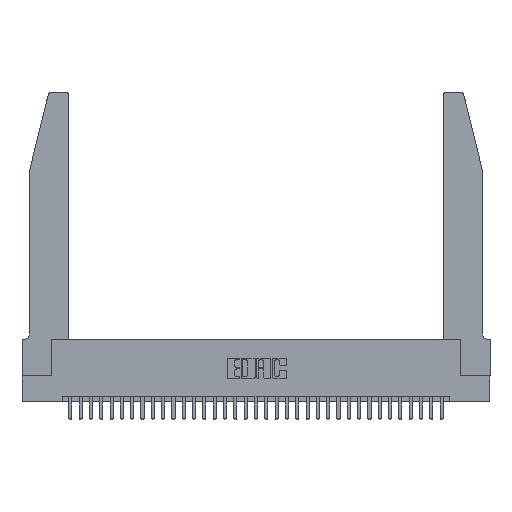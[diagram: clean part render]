
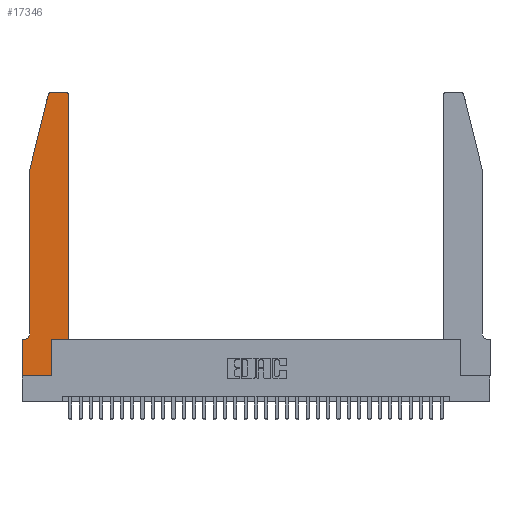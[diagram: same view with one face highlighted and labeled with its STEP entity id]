
A CAD part, top view. The second image highlights one B-rep face of the part: STEP entity #17346.
In plain terms, the highlighted planar face has unit normal (0, 0, 1).
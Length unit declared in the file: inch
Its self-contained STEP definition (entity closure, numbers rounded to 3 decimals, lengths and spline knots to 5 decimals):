
#18 = LINE ( 'NONE', #7296, #27140 ) ;
#50 = AXIS2_PLACEMENT_3D ( 'NONE', #32240, #16241, #21627 ) ;
#157 = CARTESIAN_POINT ( 'NONE',  ( 0.4505, 2.72, 0.37 ) ) ;
#393 = EDGE_LOOP ( 'NONE', ( #25358, #10739, #2610, #29178, #9738, #2797, #30110, #21953, #15608, #13104, #11026, #16467 ) ) ;
#532 = CARTESIAN_POINT ( 'NONE',  ( 0., 0., 0.37 ) ) ;
#1528 = CARTESIAN_POINT ( 'NONE',  ( 0.4205, 2.75, 0.37 ) ) ;
#1708 = EDGE_CURVE ( 'NONE', #29478, #9173, #33890, .T. ) ;
#2610 = ORIENTED_EDGE ( 'NONE', *, *, #3588, .T. ) ;
#2797 = ORIENTED_EDGE ( 'NONE', *, *, #6301, .T. ) ;
#2839 = VECTOR ( 'NONE', #18479, 39.37008 ) ;
#3296 = VECTOR ( 'NONE', #26003, 39.37008 ) ;
#3483 = EDGE_CURVE ( 'NONE', #32166, #7659, #15396, .T. ) ;
#3588 = EDGE_CURVE ( 'NONE', #21038, #27131, #17915, .T. ) ;
#3606 = VERTEX_POINT ( 'NONE', #157 ) ;
#3608 = DIRECTION ( 'NONE',  ( 1., 0., 0. ) ) ;
#3893 = CARTESIAN_POINT ( 'NONE',  ( 0.4505, 0.35, 0.37 ) ) ;
#5237 = AXIS2_PLACEMENT_3D ( 'NONE', #26455, #20796, #34541 ) ;
#5269 = CIRCLE ( 'NONE', #12655, 0.03 ) ;
#6301 = EDGE_CURVE ( 'NONE', #30680, #23756, #9746, .T. ) ;
#6349 = PLANE ( 'NONE',  #9147 ) ;
#7296 = CARTESIAN_POINT ( 'NONE',  ( 0., 0., 0.37 ) ) ;
#7659 = VERTEX_POINT ( 'NONE', #31072 ) ;
#8230 = LINE ( 'NONE', #12287, #31274 ) ;
#8306 = LINE ( 'NONE', #33399, #21710 ) ;
#8800 = EDGE_CURVE ( 'NONE', #9173, #21038, #5269, .T. ) ;
#9147 = AXIS2_PLACEMENT_3D ( 'NONE', #22483, #11845, #14546 ) ;
#9173 = VERTEX_POINT ( 'NONE', #15571 ) ;
#9477 = CARTESIAN_POINT ( 'NONE',  ( 0.0755, 2., 0.37 ) ) ;
#9738 = ORIENTED_EDGE ( 'NONE', *, *, #21469, .T. ) ;
#9746 = LINE ( 'NONE', #30534, #12687 ) ;
#9752 = CARTESIAN_POINT ( 'NONE',  ( 0.2865, 0.35, 0.37 ) ) ;
#10739 = ORIENTED_EDGE ( 'NONE', *, *, #8800, .T. ) ;
#10910 = CIRCLE ( 'NONE', #50, 0.03 ) ;
#10980 = CARTESIAN_POINT ( 'NONE',  ( 0.0755, 0.42, 0.37 ) ) ;
#11026 = ORIENTED_EDGE ( 'NONE', *, *, #15504, .T. ) ;
#11180 = CARTESIAN_POINT ( 'NONE',  ( 0.4505, 0.35, 0.37 ) ) ;
#11372 = LINE ( 'NONE', #11180, #33586 ) ;
#11845 = DIRECTION ( 'NONE',  ( 0., 0., 1. ) ) ;
#12050 = DIRECTION ( 'NONE',  ( 0., -1., 0. ) ) ;
#12287 = CARTESIAN_POINT ( 'NONE',  ( 0.0755, 2., 0.37 ) ) ;
#12655 = AXIS2_PLACEMENT_3D ( 'NONE', #27815, #22693, #22561 ) ;
#12687 = VECTOR ( 'NONE', #32031, 39.37008 ) ;
#12818 = EDGE_CURVE ( 'NONE', #23756, #34601, #18, .T. ) ;
#13095 = CARTESIAN_POINT ( 'NONE',  ( 0.2865, 0., 0.37 ) ) ;
#13104 = ORIENTED_EDGE ( 'NONE', *, *, #18372, .T. ) ;
#14381 = FACE_OUTER_BOUND ( 'NONE', #393, .T. ) ;
#14546 = DIRECTION ( 'NONE',  ( 1., 0., 0. ) ) ;
#15038 = EDGE_CURVE ( 'NONE', #34601, #32166, #8306, .T. ) ;
#15396 = LINE ( 'NONE', #9752, #17459 ) ;
#15504 = EDGE_CURVE ( 'NONE', #23414, #3606, #16597, .T. ) ;
#15571 = CARTESIAN_POINT ( 'NONE',  ( 0.284, 2.75, 0.37 ) ) ;
#15608 = ORIENTED_EDGE ( 'NONE', *, *, #3483, .T. ) ;
#16241 = DIRECTION ( 'NONE',  ( 0., 0., 1. ) ) ;
#16467 = ORIENTED_EDGE ( 'NONE', *, *, #32716, .T. ) ;
#16597 = LINE ( 'NONE', #3893, #34224 ) ;
#17217 = CARTESIAN_POINT ( 'NONE',  ( 0.25487, 2.72718, 0.37 ) ) ;
#17346 = ADVANCED_FACE ( 'NONE', ( #14381 ), #6349, .T. ) ;
#17459 = VECTOR ( 'NONE', #25511, 39.37008 ) ;
#17915 = LINE ( 'NONE', #34373, #2839 ) ;
#18372 = EDGE_CURVE ( 'NONE', #7659, #23414, #11372, .T. ) ;
#18479 = DIRECTION ( 'NONE',  ( -0.239, -0.971, 0. ) ) ;
#19720 = CARTESIAN_POINT ( 'NONE',  ( 0.0055, 0.35, 0.37 ) ) ;
#20796 = DIRECTION ( 'NONE',  ( 0., 0., -1. ) ) ;
#21038 = VERTEX_POINT ( 'NONE', #17217 ) ;
#21469 = EDGE_CURVE ( 'NONE', #29956, #30680, #31533, .T. ) ;
#21627 = DIRECTION ( 'NONE',  ( 1., 0., 0. ) ) ;
#21710 = VECTOR ( 'NONE', #28636, 39.37008 ) ;
#21931 = CARTESIAN_POINT ( 'NONE',  ( 0.4505, 0.35, 0.37 ) ) ;
#21953 = ORIENTED_EDGE ( 'NONE', *, *, #15038, .T. ) ;
#22483 = CARTESIAN_POINT ( 'NONE',  ( 0., 0.35, 0.37 ) ) ;
#22561 = DIRECTION ( 'NONE',  ( 1., 0., 0. ) ) ;
#22693 = DIRECTION ( 'NONE',  ( 0., 0., 1. ) ) ;
#23414 = VERTEX_POINT ( 'NONE', #21931 ) ;
#23576 = CARTESIAN_POINT ( 'NONE',  ( 0.2605, 2.75, 0.37 ) ) ;
#23756 = VERTEX_POINT ( 'NONE', #27217 ) ;
#25247 = DIRECTION ( 'NONE',  ( 0., 1., 0. ) ) ;
#25358 = ORIENTED_EDGE ( 'NONE', *, *, #1708, .T. ) ;
#25511 = DIRECTION ( 'NONE',  ( 0., 1., 0. ) ) ;
#25781 = EDGE_CURVE ( 'NONE', #27131, #29956, #8230, .T. ) ;
#26003 = DIRECTION ( 'NONE',  ( -1., 0., 0. ) ) ;
#26162 = DIRECTION ( 'NONE',  ( 0., -1., 0. ) ) ;
#26455 = CARTESIAN_POINT ( 'NONE',  ( 0.0055, 0.42, 0.37 ) ) ;
#27131 = VERTEX_POINT ( 'NONE', #9477 ) ;
#27140 = VECTOR ( 'NONE', #26162, 39.37008 ) ;
#27217 = CARTESIAN_POINT ( 'NONE',  ( 0., 0.35, 0.37 ) ) ;
#27815 = CARTESIAN_POINT ( 'NONE',  ( 0.284, 2.72, 0.37 ) ) ;
#28636 = DIRECTION ( 'NONE',  ( 1., 0., 0. ) ) ;
#29178 = ORIENTED_EDGE ( 'NONE', *, *, #25781, .T. ) ;
#29478 = VERTEX_POINT ( 'NONE', #1528 ) ;
#29956 = VERTEX_POINT ( 'NONE', #10980 ) ;
#30110 = ORIENTED_EDGE ( 'NONE', *, *, #12818, .T. ) ;
#30534 = CARTESIAN_POINT ( 'NONE',  ( 0.0755, 0.35, 0.37 ) ) ;
#30680 = VERTEX_POINT ( 'NONE', #19720 ) ;
#31072 = CARTESIAN_POINT ( 'NONE',  ( 0.2865, 0.35, 0.37 ) ) ;
#31274 = VECTOR ( 'NONE', #12050, 39.37008 ) ;
#31533 = CIRCLE ( 'NONE', #5237, 0.07 ) ;
#32031 = DIRECTION ( 'NONE',  ( -1., 0., 0. ) ) ;
#32166 = VERTEX_POINT ( 'NONE', #13095 ) ;
#32240 = CARTESIAN_POINT ( 'NONE',  ( 0.4205, 2.72, 0.37 ) ) ;
#32716 = EDGE_CURVE ( 'NONE', #3606, #29478, #10910, .T. ) ;
#33399 = CARTESIAN_POINT ( 'NONE',  ( 0., 0., 0.37 ) ) ;
#33586 = VECTOR ( 'NONE', #3608, 39.37008 ) ;
#33890 = LINE ( 'NONE', #23576, #3296 ) ;
#34224 = VECTOR ( 'NONE', #25247, 39.37008 ) ;
#34373 = CARTESIAN_POINT ( 'NONE',  ( 0.0755, 2., 0.37 ) ) ;
#34541 = DIRECTION ( 'NONE',  ( -1., 0., 0. ) ) ;
#34601 = VERTEX_POINT ( 'NONE', #532 ) ;
